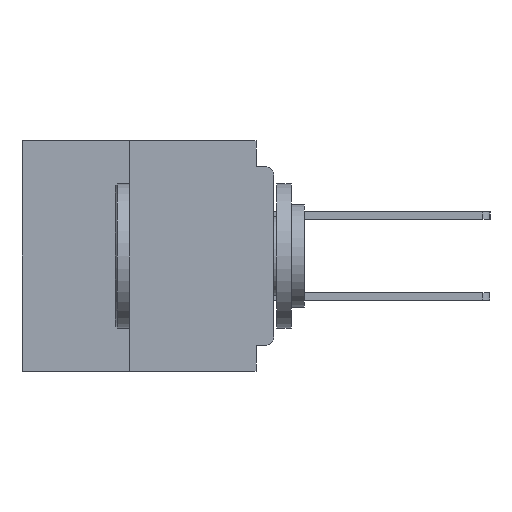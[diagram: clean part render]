
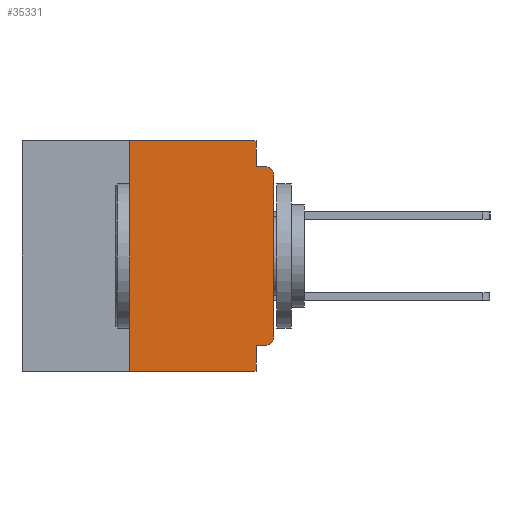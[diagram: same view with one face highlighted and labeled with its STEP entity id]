
A CAD part, left-side view. The second image highlights one B-rep face of the part: STEP entity #35331.
In plain terms, the highlighted planar face has unit normal (-1, 0, 0).
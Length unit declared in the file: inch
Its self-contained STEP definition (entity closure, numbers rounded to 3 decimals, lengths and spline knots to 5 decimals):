
#639 = CARTESIAN_POINT ( 'NONE',  ( 0., 0.015, -0.355 ) ) ;
#1892 = DIRECTION ( 'NONE',  ( 0., -1., 0. ) ) ;
#1970 = VERTEX_POINT ( 'NONE', #32614 ) ;
#2626 = ORIENTED_EDGE ( 'NONE', *, *, #8891, .F. ) ;
#2830 = FACE_OUTER_BOUND ( 'NONE', #17792, .T. ) ;
#2996 = CARTESIAN_POINT ( 'NONE',  ( 0., 0.031, -0.355 ) ) ;
#4733 = VERTEX_POINT ( 'NONE', #639 ) ;
#5420 = LINE ( 'NONE', #16445, #37458 ) ;
#6076 = EDGE_CURVE ( 'NONE', #1970, #40635, #28952, .T. ) ;
#6568 = DIRECTION ( 'NONE',  ( 0., -1., 0. ) ) ;
#7101 = VERTEX_POINT ( 'NONE', #2996 ) ;
#8365 = DIRECTION ( 'NONE',  ( 0., 0., 1. ) ) ;
#8627 = DIRECTION ( 'NONE',  ( 0., 0., -1. ) ) ;
#8884 = CARTESIAN_POINT ( 'NONE',  ( 0., 0.25, -0.4 ) ) ;
#8891 = EDGE_CURVE ( 'NONE', #33351, #29800, #29966, .T. ) ;
#9074 = EDGE_CURVE ( 'NONE', #4733, #21939, #10477, .T. ) ;
#9079 = AXIS2_PLACEMENT_3D ( 'NONE', #23673, #51617, #27729 ) ;
#9342 = CARTESIAN_POINT ( 'NONE',  ( 0., 0.437, 0. ) ) ;
#10477 = CIRCLE ( 'NONE', #50266, 0.015 ) ;
#11565 = EDGE_CURVE ( 'NONE', #15290, #29800, #20262, .T. ) ;
#12572 = VECTOR ( 'NONE', #37433, 39.37008 ) ;
#14687 = VECTOR ( 'NONE', #8627, 39.37008 ) ;
#15290 = VERTEX_POINT ( 'NONE', #22489 ) ;
#15562 = CARTESIAN_POINT ( 'NONE',  ( 0., 0., -0.34 ) ) ;
#16445 = CARTESIAN_POINT ( 'NONE',  ( 0., 0., 0. ) ) ;
#16452 = ORIENTED_EDGE ( 'NONE', *, *, #11565, .T. ) ;
#16997 = VECTOR ( 'NONE', #36989, 39.37008 ) ;
#17733 = ORIENTED_EDGE ( 'NONE', *, *, #28149, .T. ) ;
#17792 = EDGE_LOOP ( 'NONE', ( #46320, #16452, #2626, #27209, #34727, #21487, #17733, #49558, #29558, #18474 ) ) ;
#18474 = ORIENTED_EDGE ( 'NONE', *, *, #9074, .T. ) ;
#19268 = DIRECTION ( 'NONE',  ( -1., 0., 0. ) ) ;
#19914 = CARTESIAN_POINT ( 'NONE',  ( 0., 0.437, 0. ) ) ;
#20262 = CIRCLE ( 'NONE', #9079, 0.015 ) ;
#21487 = ORIENTED_EDGE ( 'NONE', *, *, #6076, .F. ) ;
#21935 = CARTESIAN_POINT ( 'NONE',  ( 0., 0., -0.045 ) ) ;
#21939 = VERTEX_POINT ( 'NONE', #15562 ) ;
#22489 = CARTESIAN_POINT ( 'NONE',  ( 0., 0., -0.06 ) ) ;
#23270 = LINE ( 'NONE', #9342, #12572 ) ;
#23673 = CARTESIAN_POINT ( 'NONE',  ( 0., 0.015, -0.06 ) ) ;
#23959 = DIRECTION ( 'NONE',  ( 0., 0., -1. ) ) ;
#25612 = LINE ( 'NONE', #35133, #45642 ) ;
#26298 = CARTESIAN_POINT ( 'NONE',  ( 0., 0.031, 0. ) ) ;
#27057 = LINE ( 'NONE', #37093, #35183 ) ;
#27209 = ORIENTED_EDGE ( 'NONE', *, *, #31550, .F. ) ;
#27442 = AXIS2_PLACEMENT_3D ( 'NONE', #19914, #47953, #23959 ) ;
#27729 = DIRECTION ( 'NONE',  ( 0., 0., -1. ) ) ;
#28149 = EDGE_CURVE ( 'NONE', #1970, #47146, #42594, .T. ) ;
#28952 = LINE ( 'NONE', #8884, #16997 ) ;
#29558 = ORIENTED_EDGE ( 'NONE', *, *, #33881, .F. ) ;
#29800 = VERTEX_POINT ( 'NONE', #41514 ) ;
#29966 = LINE ( 'NONE', #21935, #51188 ) ;
#31550 = EDGE_CURVE ( 'NONE', #37606, #33351, #36040, .T. ) ;
#31962 = CARTESIAN_POINT ( 'NONE',  ( 0., 0.031, -0.4 ) ) ;
#32614 = CARTESIAN_POINT ( 'NONE',  ( 0., 0.25, -0.4 ) ) ;
#33351 = VERTEX_POINT ( 'NONE', #36025 ) ;
#33881 = EDGE_CURVE ( 'NONE', #4733, #7101, #25612, .T. ) ;
#34727 = ORIENTED_EDGE ( 'NONE', *, *, #46704, .F. ) ;
#35133 = CARTESIAN_POINT ( 'NONE',  ( 0., 0., -0.355 ) ) ;
#35183 = VECTOR ( 'NONE', #45117, 39.37008 ) ;
#35331 = ADVANCED_FACE ( 'NONE', ( #2830 ), #43938, .F. ) ;
#36025 = CARTESIAN_POINT ( 'NONE',  ( 0., 0.031, -0.045 ) ) ;
#36040 = LINE ( 'NONE', #36392, #14687 ) ;
#36392 = CARTESIAN_POINT ( 'NONE',  ( 0., 0.031, 0. ) ) ;
#36989 = DIRECTION ( 'NONE',  ( 0., 0., 1. ) ) ;
#37093 = CARTESIAN_POINT ( 'NONE',  ( 0., 0.031, -0.4 ) ) ;
#37433 = DIRECTION ( 'NONE',  ( 0., -1., 0. ) ) ;
#37458 = VECTOR ( 'NONE', #8365, 39.37008 ) ;
#37606 = VERTEX_POINT ( 'NONE', #26298 ) ;
#38696 = CARTESIAN_POINT ( 'NONE',  ( 0., 0.437, -0.4 ) ) ;
#39163 = DIRECTION ( 'NONE',  ( 0., 1., 0. ) ) ;
#40635 = VERTEX_POINT ( 'NONE', #43313 ) ;
#41514 = CARTESIAN_POINT ( 'NONE',  ( 0., 0.015, -0.045 ) ) ;
#42594 = LINE ( 'NONE', #38696, #43594 ) ;
#43294 = CARTESIAN_POINT ( 'NONE',  ( 0., 0.015, -0.34 ) ) ;
#43313 = CARTESIAN_POINT ( 'NONE',  ( 0., 0.25, 0. ) ) ;
#43594 = VECTOR ( 'NONE', #6568, 39.37008 ) ;
#43938 = PLANE ( 'NONE',  #27442 ) ;
#45117 = DIRECTION ( 'NONE',  ( 0., 0., -1. ) ) ;
#45642 = VECTOR ( 'NONE', #39163, 39.37008 ) ;
#46320 = ORIENTED_EDGE ( 'NONE', *, *, #48868, .T. ) ;
#46689 = EDGE_CURVE ( 'NONE', #7101, #47146, #27057, .T. ) ;
#46704 = EDGE_CURVE ( 'NONE', #40635, #37606, #23270, .T. ) ;
#47146 = VERTEX_POINT ( 'NONE', #31962 ) ;
#47321 = DIRECTION ( 'NONE',  ( 0., 0., -1. ) ) ;
#47953 = DIRECTION ( 'NONE',  ( 1., 0., 0. ) ) ;
#48868 = EDGE_CURVE ( 'NONE', #21939, #15290, #5420, .T. ) ;
#49558 = ORIENTED_EDGE ( 'NONE', *, *, #46689, .F. ) ;
#50266 = AXIS2_PLACEMENT_3D ( 'NONE', #43294, #19268, #47321 ) ;
#51188 = VECTOR ( 'NONE', #1892, 39.37008 ) ;
#51617 = DIRECTION ( 'NONE',  ( -1., 0., 0. ) ) ;
